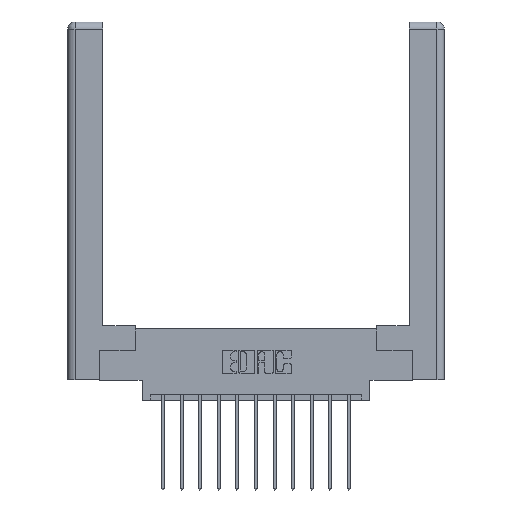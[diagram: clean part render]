
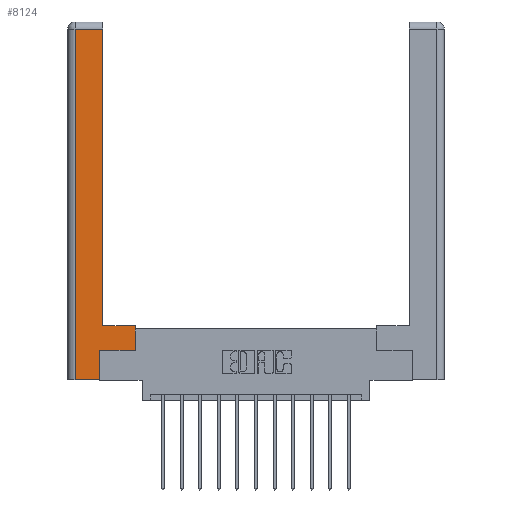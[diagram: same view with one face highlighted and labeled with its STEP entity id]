
A CAD part, top view. The second image highlights one B-rep face of the part: STEP entity #8124.
In plain terms, the highlighted planar face has unit normal (0, 0, 1).
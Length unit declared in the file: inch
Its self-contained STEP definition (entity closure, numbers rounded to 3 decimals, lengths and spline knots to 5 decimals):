
#386 = ORIENTED_EDGE ( 'NONE', *, *, #8540, .T. ) ;
#503 = CARTESIAN_POINT ( 'NONE',  ( 0.265, 0., 0. ) ) ;
#628 = EDGE_CURVE ( 'NONE', #1486, #11915, #12565, .T. ) ;
#1048 = VERTEX_POINT ( 'NONE', #3435 ) ;
#1058 = EDGE_LOOP ( 'NONE', ( #13744, #6317, #12978, #8088, #386, #4472, #10172, #8349 ) ) ;
#1235 = CARTESIAN_POINT ( 'NONE',  ( 0.0615, 2.94, 0. ) ) ;
#1486 = VERTEX_POINT ( 'NONE', #8702 ) ;
#1544 = CARTESIAN_POINT ( 'NONE',  ( 0.295, 3., 0. ) ) ;
#1567 = PLANE ( 'NONE',  #13025 ) ;
#1617 = DIRECTION ( 'NONE',  ( 0., 0., -1. ) ) ;
#2043 = EDGE_CURVE ( 'NONE', #8051, #1048, #15165, .T. ) ;
#2147 = CARTESIAN_POINT ( 'NONE',  ( 0.295, 2.94, 0. ) ) ;
#2339 = CARTESIAN_POINT ( 'NONE',  ( 0.265, 0.245, 0. ) ) ;
#2431 = VERTEX_POINT ( 'NONE', #10124 ) ;
#2504 = VERTEX_POINT ( 'NONE', #2147 ) ;
#2917 = CARTESIAN_POINT ( 'NONE',  ( 0.265, 0., 0. ) ) ;
#3335 = DIRECTION ( 'NONE',  ( 0., 1., 0. ) ) ;
#3435 = CARTESIAN_POINT ( 'NONE',  ( 0.565, 0.45, 0. ) ) ;
#3844 = LINE ( 'NONE', #9311, #7909 ) ;
#3935 = CARTESIAN_POINT ( 'NONE',  ( 0.565, 0.245, 0. ) ) ;
#4472 = ORIENTED_EDGE ( 'NONE', *, *, #7941, .T. ) ;
#4772 = EDGE_CURVE ( 'NONE', #2431, #2504, #13805, .T. ) ;
#4967 = VECTOR ( 'NONE', #7859, 39.37008 ) ;
#5125 = EDGE_CURVE ( 'NONE', #2504, #13616, #7633, .T. ) ;
#5236 = VECTOR ( 'NONE', #6254, 39.37008 ) ;
#5724 = LINE ( 'NONE', #12718, #7748 ) ;
#6254 = DIRECTION ( 'NONE',  ( 0., 1., 0. ) ) ;
#6317 = ORIENTED_EDGE ( 'NONE', *, *, #5125, .T. ) ;
#6613 = VECTOR ( 'NONE', #3335, 39.37008 ) ;
#6730 = CARTESIAN_POINT ( 'NONE',  ( 0.0615, 0., 0. ) ) ;
#7373 = EDGE_CURVE ( 'NONE', #1048, #2431, #5724, .T. ) ;
#7415 = DIRECTION ( 'NONE',  ( -1., 0., 0. ) ) ;
#7633 = LINE ( 'NONE', #1235, #11708 ) ;
#7748 = VECTOR ( 'NONE', #8939, 39.37008 ) ;
#7859 = DIRECTION ( 'NONE',  ( 0., -1., 0. ) ) ;
#7909 = VECTOR ( 'NONE', #15328, 39.37008 ) ;
#7941 = EDGE_CURVE ( 'NONE', #14470, #8051, #3844, .T. ) ;
#8051 = VERTEX_POINT ( 'NONE', #3935 ) ;
#8088 = ORIENTED_EDGE ( 'NONE', *, *, #628, .T. ) ;
#8121 = CARTESIAN_POINT ( 'NONE',  ( 0.265, 0.245, 0. ) ) ;
#8124 = ADVANCED_FACE ( 'NONE', ( #9015 ), #1567, .F. ) ;
#8135 = VECTOR ( 'NONE', #11173, 39.37008 ) ;
#8349 = ORIENTED_EDGE ( 'NONE', *, *, #7373, .T. ) ;
#8540 = EDGE_CURVE ( 'NONE', #11915, #14470, #11228, .T. ) ;
#8685 = CARTESIAN_POINT ( 'NONE',  ( 0., 0., 0. ) ) ;
#8702 = CARTESIAN_POINT ( 'NONE',  ( 0.0615, 0., 0. ) ) ;
#8939 = DIRECTION ( 'NONE',  ( -1., 0., 0. ) ) ;
#9015 = FACE_OUTER_BOUND ( 'NONE', #1058, .T. ) ;
#9311 = CARTESIAN_POINT ( 'NONE',  ( 0.565, 0.245, 0. ) ) ;
#10124 = CARTESIAN_POINT ( 'NONE',  ( 0.295, 0.45, 0. ) ) ;
#10172 = ORIENTED_EDGE ( 'NONE', *, *, #2043, .T. ) ;
#11173 = DIRECTION ( 'NONE',  ( 1., 0., 0. ) ) ;
#11228 = LINE ( 'NONE', #2339, #6613 ) ;
#11489 = DIRECTION ( 'NONE',  ( 0., 1., 0. ) ) ;
#11633 = VECTOR ( 'NONE', #11489, 39.37008 ) ;
#11685 = CARTESIAN_POINT ( 'NONE',  ( 0.0615, 2.94, 0. ) ) ;
#11708 = VECTOR ( 'NONE', #11730, 39.37008 ) ;
#11730 = DIRECTION ( 'NONE',  ( -1., 0., 0. ) ) ;
#11915 = VERTEX_POINT ( 'NONE', #503 ) ;
#12565 = LINE ( 'NONE', #2917, #8135 ) ;
#12616 = CARTESIAN_POINT ( 'NONE',  ( 0.565, 0.45, 0. ) ) ;
#12718 = CARTESIAN_POINT ( 'NONE',  ( 0.295, 0.45, 0. ) ) ;
#12978 = ORIENTED_EDGE ( 'NONE', *, *, #13520, .T. ) ;
#13025 = AXIS2_PLACEMENT_3D ( 'NONE', #8685, #1617, #7415 ) ;
#13520 = EDGE_CURVE ( 'NONE', #13616, #1486, #14628, .T. ) ;
#13616 = VERTEX_POINT ( 'NONE', #11685 ) ;
#13744 = ORIENTED_EDGE ( 'NONE', *, *, #4772, .T. ) ;
#13805 = LINE ( 'NONE', #1544, #5236 ) ;
#14470 = VERTEX_POINT ( 'NONE', #8121 ) ;
#14628 = LINE ( 'NONE', #6730, #4967 ) ;
#15165 = LINE ( 'NONE', #12616, #11633 ) ;
#15328 = DIRECTION ( 'NONE',  ( 1., 0., 0. ) ) ;
